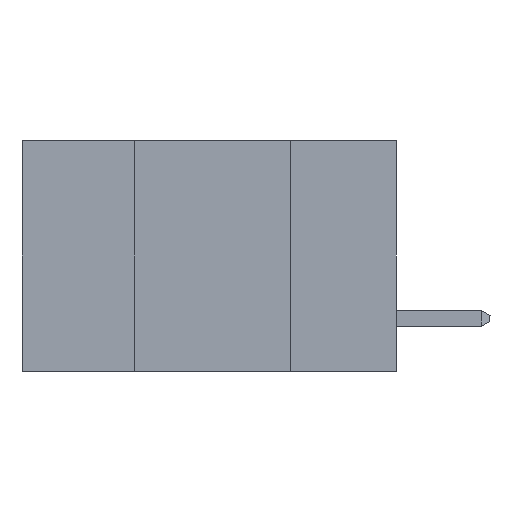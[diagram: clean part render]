
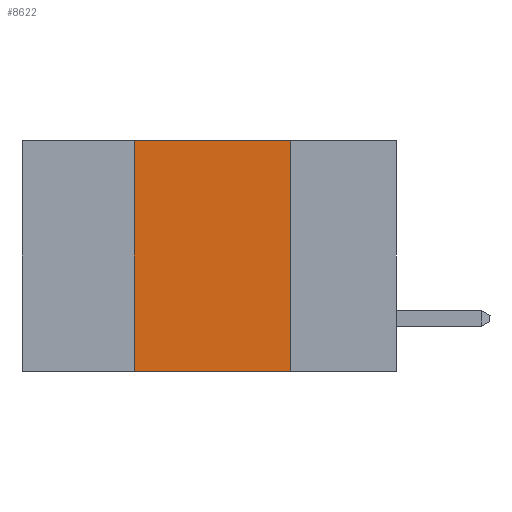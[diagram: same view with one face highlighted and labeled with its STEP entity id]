
A CAD part, left-side view. The second image highlights one B-rep face of the part: STEP entity #8622.
In plain terms, the highlighted planar face has unit normal (-1, 0, 0).
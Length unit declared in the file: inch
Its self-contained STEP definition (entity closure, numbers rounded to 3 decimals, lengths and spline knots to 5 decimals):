
#73 = ORIENTED_EDGE ( 'NONE', *, *, #4543, .T. ) ;
#102 = DIRECTION ( 'NONE',  ( 1., 0., 0. ) ) ;
#236 = VERTEX_POINT ( 'NONE', #4153 ) ;
#240 = FACE_OUTER_BOUND ( 'NONE', #839, .T. ) ;
#839 = EDGE_LOOP ( 'NONE', ( #7988, #2664, #3895, #73 ) ) ;
#2003 = VERTEX_POINT ( 'NONE', #5301 ) ;
#2435 = CARTESIAN_POINT ( 'NONE',  ( 0., 0.6, 0. ) ) ;
#2528 = CARTESIAN_POINT ( 'NONE',  ( 0., 0.42, -0.37 ) ) ;
#2664 = ORIENTED_EDGE ( 'NONE', *, *, #4484, .F. ) ;
#3296 = CARTESIAN_POINT ( 'NONE',  ( 0., 0.42, -0.37 ) ) ;
#3326 = PLANE ( 'NONE',  #8899 ) ;
#3895 = ORIENTED_EDGE ( 'NONE', *, *, #7975, .F. ) ;
#4027 = DIRECTION ( 'NONE',  ( 0., 0., -1. ) ) ;
#4153 = CARTESIAN_POINT ( 'NONE',  ( 0., 0.42, 0. ) ) ;
#4484 = EDGE_CURVE ( 'NONE', #236, #9167, #7983, .T. ) ;
#4543 = EDGE_CURVE ( 'NONE', #8605, #2003, #5477, .T. ) ;
#4657 = VECTOR ( 'NONE', #7980, 39.37008 ) ;
#5178 = VECTOR ( 'NONE', #4027, 39.37008 ) ;
#5301 = CARTESIAN_POINT ( 'NONE',  ( 0., 0.17, -0.37 ) ) ;
#5477 = LINE ( 'NONE', #8484, #9561 ) ;
#5655 = LINE ( 'NONE', #2528, #4657 ) ;
#5690 = DIRECTION ( 'NONE',  ( 0., 0., -1. ) ) ;
#5951 = VECTOR ( 'NONE', #8760, 39.37008 ) ;
#6812 = EDGE_CURVE ( 'NONE', #9167, #2003, #7220, .T. ) ;
#7220 = LINE ( 'NONE', #10152, #5178 ) ;
#7975 = EDGE_CURVE ( 'NONE', #8605, #236, #5655, .T. ) ;
#7980 = DIRECTION ( 'NONE',  ( 0., 0., 1. ) ) ;
#7983 = LINE ( 'NONE', #8832, #5951 ) ;
#7988 = ORIENTED_EDGE ( 'NONE', *, *, #6812, .F. ) ;
#8484 = CARTESIAN_POINT ( 'NONE',  ( 0., 0.6, -0.37 ) ) ;
#8603 = DIRECTION ( 'NONE',  ( 0., -1., 0. ) ) ;
#8605 = VERTEX_POINT ( 'NONE', #3296 ) ;
#8622 = ADVANCED_FACE ( 'NONE', ( #240 ), #3326, .F. ) ;
#8760 = DIRECTION ( 'NONE',  ( 0., -1., 0. ) ) ;
#8832 = CARTESIAN_POINT ( 'NONE',  ( 0., 0.6, 0. ) ) ;
#8899 = AXIS2_PLACEMENT_3D ( 'NONE', #2435, #102, #5690 ) ;
#9167 = VERTEX_POINT ( 'NONE', #10160 ) ;
#9561 = VECTOR ( 'NONE', #8603, 39.37008 ) ;
#10152 = CARTESIAN_POINT ( 'NONE',  ( 0., 0.17, -0.37 ) ) ;
#10160 = CARTESIAN_POINT ( 'NONE',  ( 0., 0.17, 0. ) ) ;
